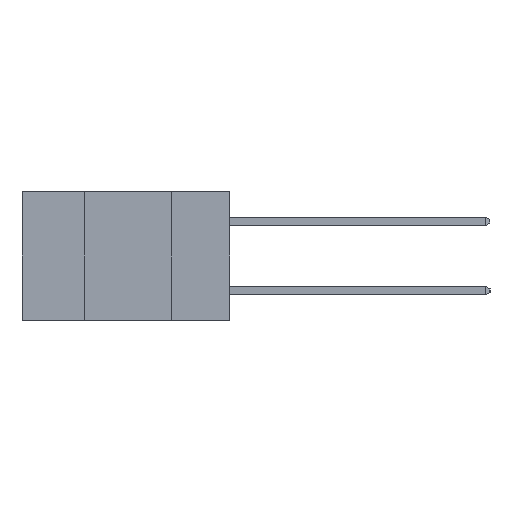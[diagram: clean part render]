
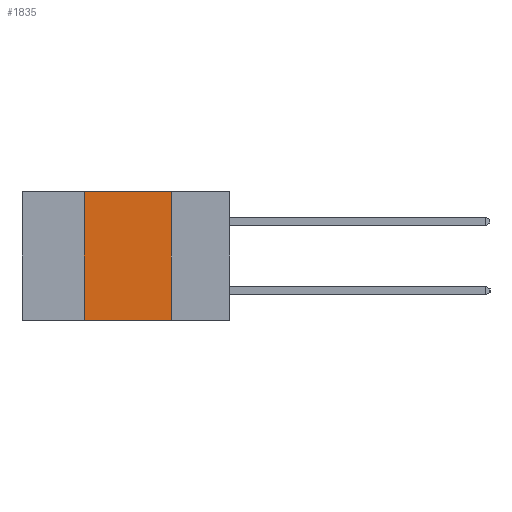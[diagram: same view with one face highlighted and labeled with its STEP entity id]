
A CAD part, left-side view. The second image highlights one B-rep face of the part: STEP entity #1835.
In plain terms, the highlighted planar face has unit normal (-1, 0, 0).
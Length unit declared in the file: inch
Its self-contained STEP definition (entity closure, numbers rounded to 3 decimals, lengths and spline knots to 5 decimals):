
#590 = LINE ( 'NONE', #5826, #7279 ) ;
#1628 = CARTESIAN_POINT ( 'NONE',  ( 0., 0.6, -0.37 ) ) ;
#1809 = ORIENTED_EDGE ( 'NONE', *, *, #9679, .T. ) ;
#1835 = ADVANCED_FACE ( 'NONE', ( #9200 ), #9943, .F. ) ;
#1956 = LINE ( 'NONE', #1628, #2810 ) ;
#2052 = CARTESIAN_POINT ( 'NONE',  ( 0., 0.6, 0. ) ) ;
#2523 = EDGE_CURVE ( 'NONE', #6887, #5216, #11159, .T. ) ;
#2694 = DIRECTION ( 'NONE',  ( 0., -1., 0. ) ) ;
#2810 = VECTOR ( 'NONE', #10714, 39.37008 ) ;
#3567 = CARTESIAN_POINT ( 'NONE',  ( 0., 0.17, -0.37 ) ) ;
#4055 = ORIENTED_EDGE ( 'NONE', *, *, #2523, .F. ) ;
#4803 = VERTEX_POINT ( 'NONE', #11096 ) ;
#4913 = AXIS2_PLACEMENT_3D ( 'NONE', #2052, #5385, #6726 ) ;
#5216 = VERTEX_POINT ( 'NONE', #9151 ) ;
#5385 = DIRECTION ( 'NONE',  ( 1., 0., 0. ) ) ;
#5455 = EDGE_CURVE ( 'NONE', #5216, #4803, #590, .T. ) ;
#5622 = ORIENTED_EDGE ( 'NONE', *, *, #5455, .F. ) ;
#5624 = LINE ( 'NONE', #10670, #10220 ) ;
#5826 = CARTESIAN_POINT ( 'NONE',  ( 0., 0.6, 0. ) ) ;
#6504 = EDGE_LOOP ( 'NONE', ( #9653, #5622, #4055, #1809 ) ) ;
#6625 = CARTESIAN_POINT ( 'NONE',  ( 0., 0.42, -0.37 ) ) ;
#6726 = DIRECTION ( 'NONE',  ( 0., 0., -1. ) ) ;
#6815 = DIRECTION ( 'NONE',  ( 0., 0., 1. ) ) ;
#6887 = VERTEX_POINT ( 'NONE', #6625 ) ;
#7279 = VECTOR ( 'NONE', #2694, 39.37008 ) ;
#7848 = VERTEX_POINT ( 'NONE', #3567 ) ;
#9151 = CARTESIAN_POINT ( 'NONE',  ( 0., 0.42, 0. ) ) ;
#9200 = FACE_OUTER_BOUND ( 'NONE', #6504, .T. ) ;
#9653 = ORIENTED_EDGE ( 'NONE', *, *, #10246, .F. ) ;
#9679 = EDGE_CURVE ( 'NONE', #6887, #7848, #1956, .T. ) ;
#9862 = CARTESIAN_POINT ( 'NONE',  ( 0., 0.42, -0.37 ) ) ;
#9943 = PLANE ( 'NONE',  #4913 ) ;
#10220 = VECTOR ( 'NONE', #11573, 39.37008 ) ;
#10246 = EDGE_CURVE ( 'NONE', #4803, #7848, #5624, .T. ) ;
#10670 = CARTESIAN_POINT ( 'NONE',  ( 0., 0.17, -0.37 ) ) ;
#10714 = DIRECTION ( 'NONE',  ( 0., -1., 0. ) ) ;
#10883 = VECTOR ( 'NONE', #6815, 39.37008 ) ;
#11096 = CARTESIAN_POINT ( 'NONE',  ( 0., 0.17, 0. ) ) ;
#11159 = LINE ( 'NONE', #9862, #10883 ) ;
#11573 = DIRECTION ( 'NONE',  ( 0., 0., -1. ) ) ;
